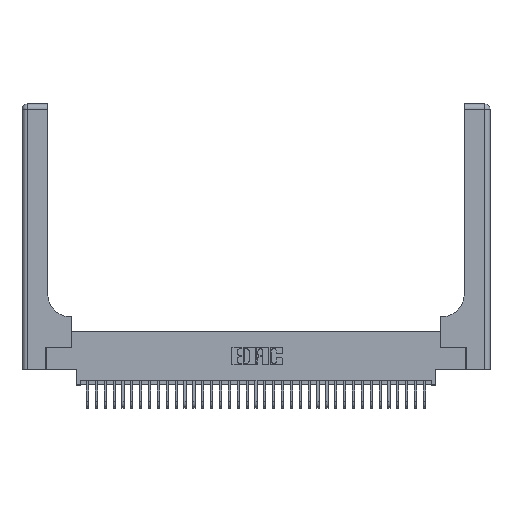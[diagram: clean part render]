
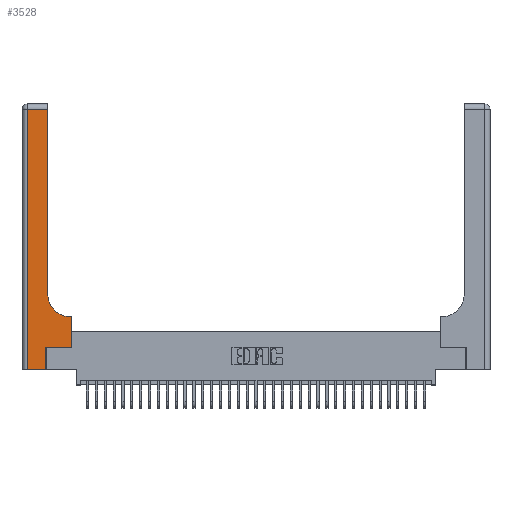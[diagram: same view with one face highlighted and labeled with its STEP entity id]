
A CAD part, top view. The second image highlights one B-rep face of the part: STEP entity #3528.
In plain terms, the highlighted planar face has unit normal (0, 0, 1).
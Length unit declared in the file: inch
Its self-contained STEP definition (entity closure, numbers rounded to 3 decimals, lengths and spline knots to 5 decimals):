
#97 = LINE ( 'NONE', #465, #30472 ) ;
#465 = CARTESIAN_POINT ( 'NONE',  ( 0.5585, 0.25, 0.37 ) ) ;
#1236 = ORIENTED_EDGE ( 'NONE', *, *, #26217, .T. ) ;
#1709 = EDGE_CURVE ( 'NONE', #34282, #3005, #97, .T. ) ;
#1943 = LINE ( 'NONE', #12863, #2870 ) ;
#2870 = VECTOR ( 'NONE', #21680, 39.37008 ) ;
#2960 = DIRECTION ( 'NONE',  ( -1., 0., 0. ) ) ;
#3005 = VERTEX_POINT ( 'NONE', #32458 ) ;
#3528 = ADVANCED_FACE ( 'NONE', ( #34490 ), #14734, .F. ) ;
#3629 = ORIENTED_EDGE ( 'NONE', *, *, #22125, .T. ) ;
#4043 = AXIS2_PLACEMENT_3D ( 'NONE', #17484, #37829, #20432 ) ;
#4196 = EDGE_CURVE ( 'NONE', #3005, #21116, #12591, .T. ) ;
#5205 = CARTESIAN_POINT ( 'NONE',  ( 0.269, 0., 0.37 ) ) ;
#5538 = DIRECTION ( 'NONE',  ( -1., 0., 0. ) ) ;
#5741 = CARTESIAN_POINT ( 'NONE',  ( 0.269, 0.25, 0.37 ) ) ;
#5863 = CARTESIAN_POINT ( 'NONE',  ( 0.5415, 0.6, 0.37 ) ) ;
#5895 = CARTESIAN_POINT ( 'NONE',  ( 0.5585, 0.25, 0.37 ) ) ;
#5986 = EDGE_CURVE ( 'NONE', #34543, #13758, #37515, .T. ) ;
#7749 = LINE ( 'NONE', #13681, #21530 ) ;
#8638 = EDGE_CURVE ( 'NONE', #12390, #17321, #13294, .T. ) ;
#8806 = DIRECTION ( 'NONE',  ( 0., 1., 0. ) ) ;
#9671 = ORIENTED_EDGE ( 'NONE', *, *, #14788, .T. ) ;
#12359 = VERTEX_POINT ( 'NONE', #26968 ) ;
#12390 = VERTEX_POINT ( 'NONE', #30008 ) ;
#12591 = LINE ( 'NONE', #28983, #34890 ) ;
#12863 = CARTESIAN_POINT ( 'NONE',  ( 0.269, 0.25, 0.37 ) ) ;
#13115 = CARTESIAN_POINT ( 'NONE',  ( 0., 0., 0.37 ) ) ;
#13294 = LINE ( 'NONE', #14700, #27865 ) ;
#13681 = CARTESIAN_POINT ( 'NONE',  ( 0., 2.94, 0.37 ) ) ;
#13758 = VERTEX_POINT ( 'NONE', #17583 ) ;
#14700 = CARTESIAN_POINT ( 'NONE',  ( 0.2915, 3., 0.37 ) ) ;
#14734 = PLANE ( 'NONE',  #36627 ) ;
#14788 = EDGE_CURVE ( 'NONE', #17321, #34543, #7749, .T. ) ;
#15786 = EDGE_CURVE ( 'NONE', #12359, #19110, #35061, .T. ) ;
#16610 = DIRECTION ( 'NONE',  ( -1., 0., 0. ) ) ;
#17321 = VERTEX_POINT ( 'NONE', #36072 ) ;
#17390 = ORIENTED_EDGE ( 'NONE', *, *, #5986, .T. ) ;
#17484 = CARTESIAN_POINT ( 'NONE',  ( 0.5415, 0.85, 0.37 ) ) ;
#17583 = CARTESIAN_POINT ( 'NONE',  ( 0.06, 0., 0.37 ) ) ;
#17692 = CARTESIAN_POINT ( 'NONE',  ( 0., 3., 0.37 ) ) ;
#18683 = EDGE_LOOP ( 'NONE', ( #22556, #9671, #17390, #3629, #28854, #23533, #28244, #19001, #1236 ) ) ;
#19001 = ORIENTED_EDGE ( 'NONE', *, *, #4196, .T. ) ;
#19110 = VERTEX_POINT ( 'NONE', #5741 ) ;
#19467 = CARTESIAN_POINT ( 'NONE',  ( 0.06, 3., 0.37 ) ) ;
#20432 = DIRECTION ( 'NONE',  ( 1., 0., 0. ) ) ;
#20632 = DIRECTION ( 'NONE',  ( 0., 0., -1. ) ) ;
#21116 = VERTEX_POINT ( 'NONE', #5863 ) ;
#21530 = VECTOR ( 'NONE', #16610, 39.37008 ) ;
#21680 = DIRECTION ( 'NONE',  ( 1., 0., 0. ) ) ;
#22125 = EDGE_CURVE ( 'NONE', #13758, #12359, #32402, .T. ) ;
#22556 = ORIENTED_EDGE ( 'NONE', *, *, #8638, .T. ) ;
#22986 = VECTOR ( 'NONE', #36876, 39.37008 ) ;
#23533 = ORIENTED_EDGE ( 'NONE', *, *, #36185, .T. ) ;
#23985 = CIRCLE ( 'NONE', #4043, 0.25 ) ;
#26217 = EDGE_CURVE ( 'NONE', #21116, #12390, #23985, .T. ) ;
#26968 = CARTESIAN_POINT ( 'NONE',  ( 0.269, 0., 0.37 ) ) ;
#26980 = DIRECTION ( 'NONE',  ( 0., 1., 0. ) ) ;
#27345 = VECTOR ( 'NONE', #31701, 39.37008 ) ;
#27416 = CARTESIAN_POINT ( 'NONE',  ( 0.06, 2.94, 0.37 ) ) ;
#27865 = VECTOR ( 'NONE', #8806, 39.37008 ) ;
#28244 = ORIENTED_EDGE ( 'NONE', *, *, #1709, .T. ) ;
#28854 = ORIENTED_EDGE ( 'NONE', *, *, #15786, .T. ) ;
#28983 = CARTESIAN_POINT ( 'NONE',  ( 0.2915, 0.6, 0.37 ) ) ;
#30008 = CARTESIAN_POINT ( 'NONE',  ( 0.2915, 0.85, 0.37 ) ) ;
#30472 = VECTOR ( 'NONE', #26980, 39.37008 ) ;
#30551 = DIRECTION ( 'NONE',  ( 1., 0., 0. ) ) ;
#31503 = VECTOR ( 'NONE', #30551, 39.37008 ) ;
#31701 = DIRECTION ( 'NONE',  ( 0., 1., 0. ) ) ;
#32402 = LINE ( 'NONE', #13115, #31503 ) ;
#32458 = CARTESIAN_POINT ( 'NONE',  ( 0.5585, 0.6, 0.37 ) ) ;
#34282 = VERTEX_POINT ( 'NONE', #5895 ) ;
#34490 = FACE_OUTER_BOUND ( 'NONE', #18683, .T. ) ;
#34543 = VERTEX_POINT ( 'NONE', #27416 ) ;
#34890 = VECTOR ( 'NONE', #5538, 39.37008 ) ;
#35061 = LINE ( 'NONE', #5205, #27345 ) ;
#36072 = CARTESIAN_POINT ( 'NONE',  ( 0.2915, 2.94, 0.37 ) ) ;
#36185 = EDGE_CURVE ( 'NONE', #19110, #34282, #1943, .T. ) ;
#36627 = AXIS2_PLACEMENT_3D ( 'NONE', #17692, #20632, #2960 ) ;
#36876 = DIRECTION ( 'NONE',  ( 0., -1., 0. ) ) ;
#37515 = LINE ( 'NONE', #19467, #22986 ) ;
#37829 = DIRECTION ( 'NONE',  ( 0., 0., -1. ) ) ;
